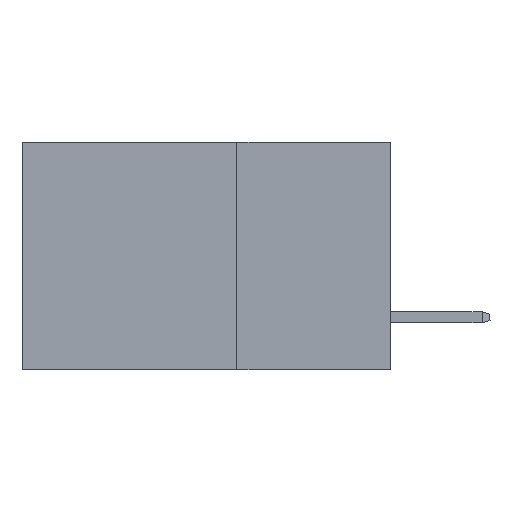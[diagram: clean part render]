
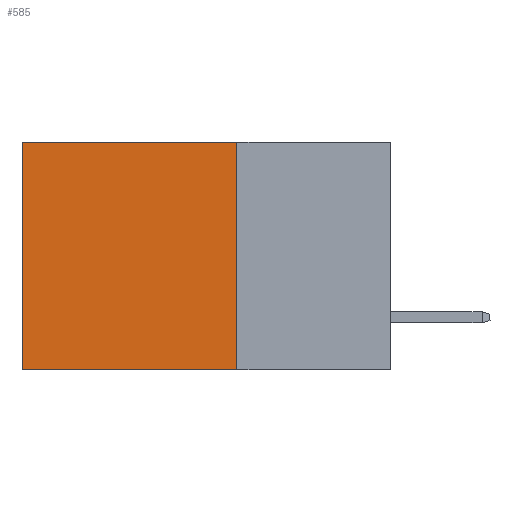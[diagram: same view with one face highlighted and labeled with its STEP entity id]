
A CAD part, left-side view. The second image highlights one B-rep face of the part: STEP entity #585.
In plain terms, the highlighted planar face has unit normal (-1, 0, 0).
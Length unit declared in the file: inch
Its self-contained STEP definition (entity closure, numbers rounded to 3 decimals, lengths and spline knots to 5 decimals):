
#581 = EDGE_CURVE ( 'NONE', #5994, #11277, #11873, .T. ) ;
#585 = ADVANCED_FACE ( 'NONE', ( #4510 ), #4392, .F. ) ;
#1050 = EDGE_LOOP ( 'NONE', ( #6891, #6934, #7066, #7173 ) ) ;
#1123 = CARTESIAN_POINT ( 'NONE',  ( 0.2875, 0.6, 0. ) ) ;
#1708 = EDGE_CURVE ( 'NONE', #11564, #11277, #4785, .T. ) ;
#2049 = EDGE_CURVE ( 'NONE', #6398, #11564, #6323, .T. ) ;
#2070 = VECTOR ( 'NONE', #8766, 39.37008 ) ;
#2181 = DIRECTION ( 'NONE',  ( 0., 0., -1. ) ) ;
#2350 = DIRECTION ( 'NONE',  ( 1., 0., 0. ) ) ;
#2435 = VECTOR ( 'NONE', #2181, 39.37008 ) ;
#2792 = DIRECTION ( 'NONE',  ( 0., 0., -1. ) ) ;
#3251 = CARTESIAN_POINT ( 'NONE',  ( 0.2875, 0.25, 0. ) ) ;
#3811 = VECTOR ( 'NONE', #8728, 39.37008 ) ;
#4392 = PLANE ( 'NONE',  #4979 ) ;
#4510 = FACE_OUTER_BOUND ( 'NONE', #1050, .T. ) ;
#4785 = LINE ( 'NONE', #8821, #2070 ) ;
#4979 = AXIS2_PLACEMENT_3D ( 'NONE', #3251, #2350, #2792 ) ;
#5700 = CARTESIAN_POINT ( 'NONE',  ( 0.2875, 0.6, -0.37 ) ) ;
#5994 = VERTEX_POINT ( 'NONE', #12085 ) ;
#6075 = CARTESIAN_POINT ( 'NONE',  ( 0.2875, 0.25, -0.37 ) ) ;
#6323 = LINE ( 'NONE', #7121, #8469 ) ;
#6398 = VERTEX_POINT ( 'NONE', #8241 ) ;
#6751 = DIRECTION ( 'NONE',  ( 0., 0., -1. ) ) ;
#6891 = ORIENTED_EDGE ( 'NONE', *, *, #581, .T. ) ;
#6934 = ORIENTED_EDGE ( 'NONE', *, *, #1708, .F. ) ;
#7066 = ORIENTED_EDGE ( 'NONE', *, *, #2049, .F. ) ;
#7103 = EDGE_CURVE ( 'NONE', #6398, #5994, #11279, .T. ) ;
#7121 = CARTESIAN_POINT ( 'NONE',  ( 0.2875, 0.25, 0. ) ) ;
#7173 = ORIENTED_EDGE ( 'NONE', *, *, #7103, .T. ) ;
#8241 = CARTESIAN_POINT ( 'NONE',  ( 0.2875, 0.25, 0. ) ) ;
#8469 = VECTOR ( 'NONE', #6751, 39.37008 ) ;
#8728 = DIRECTION ( 'NONE',  ( 0., 1., 0. ) ) ;
#8766 = DIRECTION ( 'NONE',  ( 0., 1., 0. ) ) ;
#8821 = CARTESIAN_POINT ( 'NONE',  ( 0.2875, 0.25, -0.37 ) ) ;
#11277 = VERTEX_POINT ( 'NONE', #5700 ) ;
#11279 = LINE ( 'NONE', #12278, #3811 ) ;
#11564 = VERTEX_POINT ( 'NONE', #6075 ) ;
#11873 = LINE ( 'NONE', #1123, #2435 ) ;
#12085 = CARTESIAN_POINT ( 'NONE',  ( 0.2875, 0.6, 0. ) ) ;
#12278 = CARTESIAN_POINT ( 'NONE',  ( 0.2875, 0.25, 0. ) ) ;
